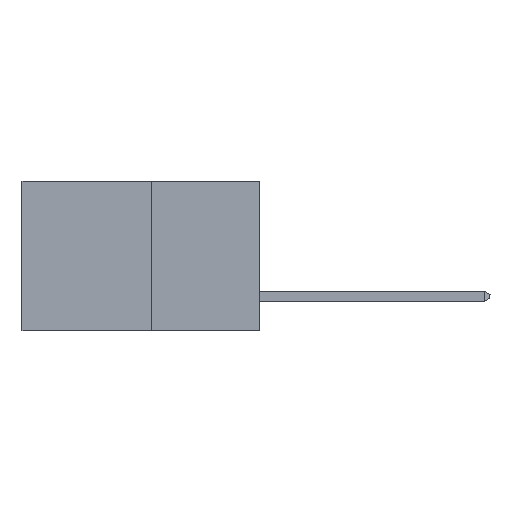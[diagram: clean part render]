
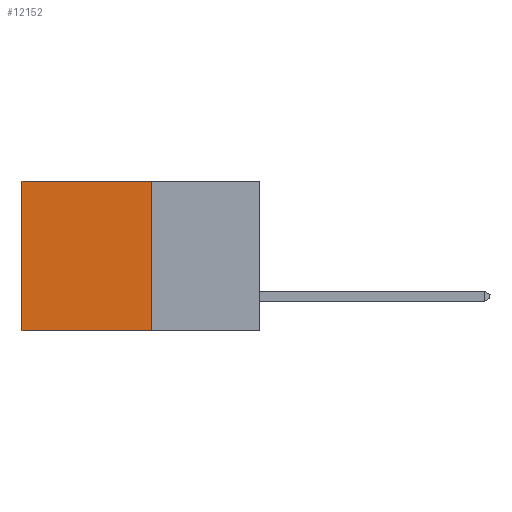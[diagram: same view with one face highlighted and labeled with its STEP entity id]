
A CAD part, left-side view. The second image highlights one B-rep face of the part: STEP entity #12152.
In plain terms, the highlighted planar face has unit normal (-1, 0, 0).
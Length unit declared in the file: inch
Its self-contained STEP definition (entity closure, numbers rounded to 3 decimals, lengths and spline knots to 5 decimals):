
#236 = ORIENTED_EDGE ( 'NONE', *, *, #3071, .F. ) ;
#318 = VERTEX_POINT ( 'NONE', #10994 ) ;
#430 = DIRECTION ( 'NONE',  ( 0., 1., 0. ) ) ;
#439 = CARTESIAN_POINT ( 'NONE',  ( 0.277, 0.59, -0.37 ) ) ;
#895 = CARTESIAN_POINT ( 'NONE',  ( 0.277, 0.27, 0. ) ) ;
#1154 = VECTOR ( 'NONE', #430, 39.37008 ) ;
#1554 = LINE ( 'NONE', #6518, #1154 ) ;
#1724 = DIRECTION ( 'NONE',  ( 0., 0., -1. ) ) ;
#2584 = LINE ( 'NONE', #6760, #5747 ) ;
#2744 = DIRECTION ( 'NONE',  ( 0., 0., -1. ) ) ;
#2851 = CARTESIAN_POINT ( 'NONE',  ( 0.277, 0.27, -0.37 ) ) ;
#3019 = LINE ( 'NONE', #2851, #11140 ) ;
#3071 = EDGE_CURVE ( 'NONE', #318, #8048, #1554, .T. ) ;
#3337 = VECTOR ( 'NONE', #1724, 39.37008 ) ;
#3803 = CARTESIAN_POINT ( 'NONE',  ( 0.277, 0.59, 0. ) ) ;
#4501 = ORIENTED_EDGE ( 'NONE', *, *, #8548, .T. ) ;
#4607 = AXIS2_PLACEMENT_3D ( 'NONE', #12758, #13851, #7143 ) ;
#5378 = VERTEX_POINT ( 'NONE', #895 ) ;
#5429 = ORIENTED_EDGE ( 'NONE', *, *, #7267, .T. ) ;
#5450 = FACE_OUTER_BOUND ( 'NONE', #12031, .T. ) ;
#5747 = VECTOR ( 'NONE', #6832, 39.37008 ) ;
#5859 = EDGE_CURVE ( 'NONE', #5378, #318, #3019, .T. ) ;
#6518 = CARTESIAN_POINT ( 'NONE',  ( 0.277, 0.27, -0.37 ) ) ;
#6760 = CARTESIAN_POINT ( 'NONE',  ( 0.277, 0.27, 0. ) ) ;
#6832 = DIRECTION ( 'NONE',  ( 0., 1., 0. ) ) ;
#7143 = DIRECTION ( 'NONE',  ( 0., 0., -1. ) ) ;
#7267 = EDGE_CURVE ( 'NONE', #5378, #10687, #2584, .T. ) ;
#8048 = VERTEX_POINT ( 'NONE', #10231 ) ;
#8548 = EDGE_CURVE ( 'NONE', #10687, #8048, #12842, .T. ) ;
#10231 = CARTESIAN_POINT ( 'NONE',  ( 0.277, 0.59, -0.37 ) ) ;
#10687 = VERTEX_POINT ( 'NONE', #3803 ) ;
#10994 = CARTESIAN_POINT ( 'NONE',  ( 0.277, 0.27, -0.37 ) ) ;
#11140 = VECTOR ( 'NONE', #2744, 39.37008 ) ;
#11660 = PLANE ( 'NONE',  #4607 ) ;
#12031 = EDGE_LOOP ( 'NONE', ( #4501, #236, #13741, #5429 ) ) ;
#12152 = ADVANCED_FACE ( 'NONE', ( #5450 ), #11660, .F. ) ;
#12758 = CARTESIAN_POINT ( 'NONE',  ( 0.277, 0.27, -0.37 ) ) ;
#12842 = LINE ( 'NONE', #439, #3337 ) ;
#13741 = ORIENTED_EDGE ( 'NONE', *, *, #5859, .F. ) ;
#13851 = DIRECTION ( 'NONE',  ( 1., 0., 0. ) ) ;
